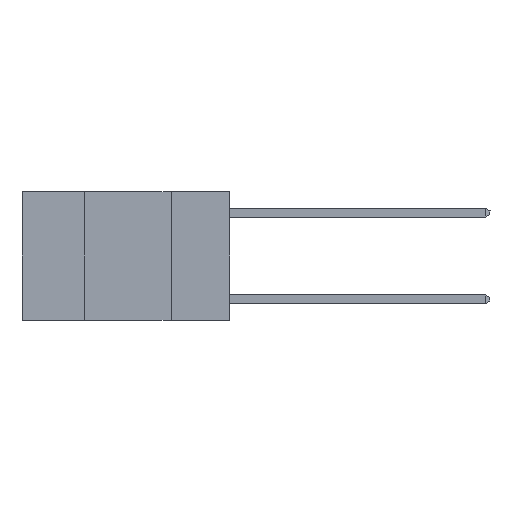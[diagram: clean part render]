
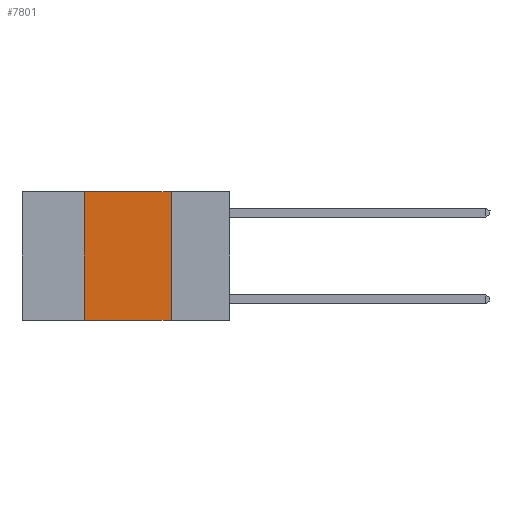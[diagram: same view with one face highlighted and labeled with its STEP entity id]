
A CAD part, left-side view. The second image highlights one B-rep face of the part: STEP entity #7801.
In plain terms, the highlighted planar face has unit normal (-1, 0, 0).
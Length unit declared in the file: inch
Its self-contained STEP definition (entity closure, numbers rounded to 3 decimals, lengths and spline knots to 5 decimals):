
#34 = CARTESIAN_POINT ( 'NONE',  ( 0., 0.17, 0. ) ) ;
#489 = PLANE ( 'NONE',  #5736 ) ;
#515 = VERTEX_POINT ( 'NONE', #4861 ) ;
#552 = EDGE_CURVE ( 'NONE', #2146, #1030, #8681, .T. ) ;
#1030 = VERTEX_POINT ( 'NONE', #5517 ) ;
#1599 = EDGE_CURVE ( 'NONE', #8354, #1030, #4615, .T. ) ;
#1655 = CARTESIAN_POINT ( 'NONE',  ( 0., 0.42, 0. ) ) ;
#2032 = EDGE_LOOP ( 'NONE', ( #7210, #7349, #5345, #10114 ) ) ;
#2146 = VERTEX_POINT ( 'NONE', #34 ) ;
#2927 = LINE ( 'NONE', #1655, #9491 ) ;
#3008 = CARTESIAN_POINT ( 'NONE',  ( 0., 0.42, -0.37 ) ) ;
#3094 = CARTESIAN_POINT ( 'NONE',  ( 0., 0.6, 0. ) ) ;
#3134 = DIRECTION ( 'NONE',  ( 1., 0., 0. ) ) ;
#3676 = CARTESIAN_POINT ( 'NONE',  ( 0., 0.6, -0.37 ) ) ;
#4071 = DIRECTION ( 'NONE',  ( 0., 0., -1. ) ) ;
#4615 = LINE ( 'NONE', #3676, #8895 ) ;
#4861 = CARTESIAN_POINT ( 'NONE',  ( 0., 0.42, 0. ) ) ;
#5205 = EDGE_CURVE ( 'NONE', #8354, #515, #2927, .T. ) ;
#5328 = FACE_OUTER_BOUND ( 'NONE', #2032, .T. ) ;
#5345 = ORIENTED_EDGE ( 'NONE', *, *, #5205, .F. ) ;
#5517 = CARTESIAN_POINT ( 'NONE',  ( 0., 0.17, -0.37 ) ) ;
#5736 = AXIS2_PLACEMENT_3D ( 'NONE', #9937, #3134, #9121 ) ;
#6303 = EDGE_CURVE ( 'NONE', #515, #2146, #7345, .T. ) ;
#6615 = CARTESIAN_POINT ( 'NONE',  ( 0., 0.17, 0. ) ) ;
#7210 = ORIENTED_EDGE ( 'NONE', *, *, #552, .F. ) ;
#7345 = LINE ( 'NONE', #3094, #9324 ) ;
#7349 = ORIENTED_EDGE ( 'NONE', *, *, #6303, .F. ) ;
#7801 = ADVANCED_FACE ( 'NONE', ( #5328 ), #489, .F. ) ;
#8354 = VERTEX_POINT ( 'NONE', #3008 ) ;
#8413 = VECTOR ( 'NONE', #4071, 39.37008 ) ;
#8681 = LINE ( 'NONE', #6615, #8413 ) ;
#8807 = DIRECTION ( 'NONE',  ( 0., -1., 0. ) ) ;
#8895 = VECTOR ( 'NONE', #8807, 39.37008 ) ;
#9121 = DIRECTION ( 'NONE',  ( 0., 0., -1. ) ) ;
#9324 = VECTOR ( 'NONE', #10793, 39.37008 ) ;
#9491 = VECTOR ( 'NONE', #10208, 39.37008 ) ;
#9937 = CARTESIAN_POINT ( 'NONE',  ( 0., 0.6, 0. ) ) ;
#10114 = ORIENTED_EDGE ( 'NONE', *, *, #1599, .T. ) ;
#10208 = DIRECTION ( 'NONE',  ( 0., 0., 1. ) ) ;
#10793 = DIRECTION ( 'NONE',  ( 0., -1., 0. ) ) ;
